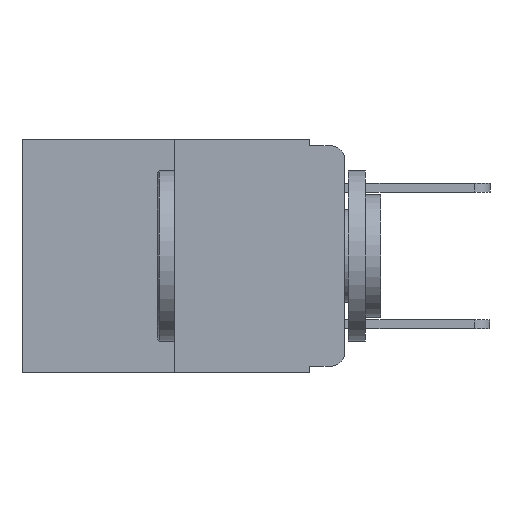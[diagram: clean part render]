
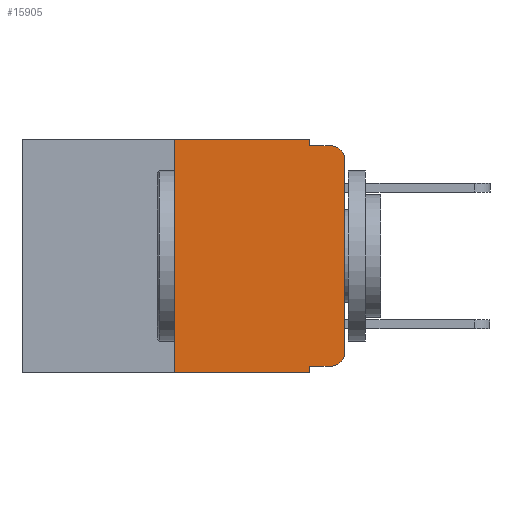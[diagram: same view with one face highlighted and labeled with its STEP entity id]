
A CAD part, left-side view. The second image highlights one B-rep face of the part: STEP entity #15905.
In plain terms, the highlighted planar face has unit normal (-1, 0, 0).
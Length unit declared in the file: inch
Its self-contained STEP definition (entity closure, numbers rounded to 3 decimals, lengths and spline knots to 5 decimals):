
#973 = CARTESIAN_POINT ( 'NONE',  ( 0., 0.473, -0.343 ) ) ;
#1327 = DIRECTION ( 'NONE',  ( 0., 0., -1. ) ) ;
#2011 = VERTEX_POINT ( 'NONE', #2766 ) ;
#2129 = PLANE ( 'NONE',  #23795 ) ;
#2137 = AXIS2_PLACEMENT_3D ( 'NONE', #9203, #22950, #11241 ) ;
#2766 = CARTESIAN_POINT ( 'NONE',  ( 0., 0.02, -0.01 ) ) ;
#2805 = EDGE_CURVE ( 'NONE', #16652, #19790, #15416, .T. ) ;
#3169 = EDGE_CURVE ( 'NONE', #7049, #22149, #18451, .T. ) ;
#3630 = CARTESIAN_POINT ( 'NONE',  ( 0., 0.02, -0.333 ) ) ;
#4014 = CARTESIAN_POINT ( 'NONE',  ( 0., 0., -0.313 ) ) ;
#4418 = CARTESIAN_POINT ( 'NONE',  ( 0., 0.25, 0. ) ) ;
#4580 = DIRECTION ( 'NONE',  ( 0., -1., 0. ) ) ;
#6301 = VECTOR ( 'NONE', #15349, 39.37008 ) ;
#6888 = ORIENTED_EDGE ( 'NONE', *, *, #8202, .T. ) ;
#7005 = AXIS2_PLACEMENT_3D ( 'NONE', #25070, #13385, #1327 ) ;
#7049 = VERTEX_POINT ( 'NONE', #14574 ) ;
#8202 = EDGE_CURVE ( 'NONE', #19790, #2011, #19039, .T. ) ;
#8248 = VERTEX_POINT ( 'NONE', #19363 ) ;
#8792 = ORIENTED_EDGE ( 'NONE', *, *, #24040, .F. ) ;
#8833 = FACE_OUTER_BOUND ( 'NONE', #12147, .T. ) ;
#9203 = CARTESIAN_POINT ( 'NONE',  ( 0., 0.02, -0.313 ) ) ;
#9620 = CARTESIAN_POINT ( 'NONE',  ( 0., 0., 0. ) ) ;
#10225 = VECTOR ( 'NONE', #24626, 39.37008 ) ;
#10376 = CARTESIAN_POINT ( 'NONE',  ( 0., 0.473, 0. ) ) ;
#10720 = VERTEX_POINT ( 'NONE', #17561 ) ;
#11211 = EDGE_CURVE ( 'NONE', #16038, #10720, #17134, .T. ) ;
#11241 = DIRECTION ( 'NONE',  ( 0., 0., -1. ) ) ;
#11682 = LINE ( 'NONE', #21275, #6301 ) ;
#11725 = DIRECTION ( 'NONE',  ( 0., -1., 0. ) ) ;
#11776 = EDGE_CURVE ( 'NONE', #17526, #10720, #19272, .T. ) ;
#12050 = CARTESIAN_POINT ( 'NONE',  ( 0., 0.051, 0. ) ) ;
#12082 = EDGE_CURVE ( 'NONE', #17526, #20220, #11682, .T. ) ;
#12147 = EDGE_LOOP ( 'NONE', ( #16150, #6888, #25046, #14344, #19563, #8792, #20488, #25660, #18972, #24186 ) ) ;
#12388 = DIRECTION ( 'NONE',  ( 0., 0., -1. ) ) ;
#12474 = LINE ( 'NONE', #12050, #16990 ) ;
#12502 = DIRECTION ( 'NONE',  ( 0., 0., 1. ) ) ;
#13066 = DIRECTION ( 'NONE',  ( 0., -1., 0. ) ) ;
#13286 = VECTOR ( 'NONE', #11725, 39.37008 ) ;
#13385 = DIRECTION ( 'NONE',  ( -1., 0., 0. ) ) ;
#13679 = CIRCLE ( 'NONE', #2137, 0.02 ) ;
#14344 = ORIENTED_EDGE ( 'NONE', *, *, #21413, .F. ) ;
#14383 = LINE ( 'NONE', #16442, #18985 ) ;
#14574 = CARTESIAN_POINT ( 'NONE',  ( 0., 0.25, 0. ) ) ;
#15349 = DIRECTION ( 'NONE',  ( 0., -1., 0. ) ) ;
#15416 = LINE ( 'NONE', #9620, #10225 ) ;
#15485 = CARTESIAN_POINT ( 'NONE',  ( 0., 0.051, 0. ) ) ;
#15905 = ADVANCED_FACE ( 'NONE', ( #8833 ), #2129, .F. ) ;
#16038 = VERTEX_POINT ( 'NONE', #18079 ) ;
#16124 = EDGE_CURVE ( 'NONE', #8248, #2011, #14383, .T. ) ;
#16150 = ORIENTED_EDGE ( 'NONE', *, *, #2805, .T. ) ;
#16442 = CARTESIAN_POINT ( 'NONE',  ( 0., 0.051, -0.01 ) ) ;
#16453 = CARTESIAN_POINT ( 'NONE',  ( 0., 0.051, 0. ) ) ;
#16652 = VERTEX_POINT ( 'NONE', #4014 ) ;
#16990 = VECTOR ( 'NONE', #17946, 39.37008 ) ;
#17134 = LINE ( 'NONE', #973, #21771 ) ;
#17526 = VERTEX_POINT ( 'NONE', #24785 ) ;
#17561 = CARTESIAN_POINT ( 'NONE',  ( 0., 0.051, -0.343 ) ) ;
#17946 = DIRECTION ( 'NONE',  ( 0., 0., -1. ) ) ;
#18079 = CARTESIAN_POINT ( 'NONE',  ( 0., 0.25, -0.343 ) ) ;
#18440 = DIRECTION ( 'NONE',  ( 0., 0., -1. ) ) ;
#18451 = LINE ( 'NONE', #25344, #13286 ) ;
#18972 = ORIENTED_EDGE ( 'NONE', *, *, #12082, .T. ) ;
#18985 = VECTOR ( 'NONE', #4580, 39.37008 ) ;
#19039 = CIRCLE ( 'NONE', #7005, 0.02 ) ;
#19272 = LINE ( 'NONE', #16453, #23877 ) ;
#19363 = CARTESIAN_POINT ( 'NONE',  ( 0., 0.051, -0.01 ) ) ;
#19563 = ORIENTED_EDGE ( 'NONE', *, *, #3169, .F. ) ;
#19790 = VERTEX_POINT ( 'NONE', #20087 ) ;
#20087 = CARTESIAN_POINT ( 'NONE',  ( 0., 0., -0.03 ) ) ;
#20220 = VERTEX_POINT ( 'NONE', #3630 ) ;
#20331 = VECTOR ( 'NONE', #12502, 39.37008 ) ;
#20488 = ORIENTED_EDGE ( 'NONE', *, *, #11211, .T. ) ;
#21275 = CARTESIAN_POINT ( 'NONE',  ( 0., 0.051, -0.333 ) ) ;
#21413 = EDGE_CURVE ( 'NONE', #22149, #8248, #12474, .T. ) ;
#21771 = VECTOR ( 'NONE', #13066, 39.37008 ) ;
#22149 = VERTEX_POINT ( 'NONE', #15485 ) ;
#22569 = EDGE_CURVE ( 'NONE', #20220, #16652, #13679, .T. ) ;
#22950 = DIRECTION ( 'NONE',  ( -1., 0., 0. ) ) ;
#23795 = AXIS2_PLACEMENT_3D ( 'NONE', #10376, #24071, #12388 ) ;
#23877 = VECTOR ( 'NONE', #18440, 39.37008 ) ;
#24040 = EDGE_CURVE ( 'NONE', #16038, #7049, #25511, .T. ) ;
#24071 = DIRECTION ( 'NONE',  ( 1., 0., 0. ) ) ;
#24186 = ORIENTED_EDGE ( 'NONE', *, *, #22569, .T. ) ;
#24626 = DIRECTION ( 'NONE',  ( 0., 0., 1. ) ) ;
#24785 = CARTESIAN_POINT ( 'NONE',  ( 0., 0.051, -0.333 ) ) ;
#25046 = ORIENTED_EDGE ( 'NONE', *, *, #16124, .F. ) ;
#25070 = CARTESIAN_POINT ( 'NONE',  ( 0., 0.02, -0.03 ) ) ;
#25344 = CARTESIAN_POINT ( 'NONE',  ( 0., 0.473, 0. ) ) ;
#25511 = LINE ( 'NONE', #4418, #20331 ) ;
#25660 = ORIENTED_EDGE ( 'NONE', *, *, #11776, .F. ) ;
